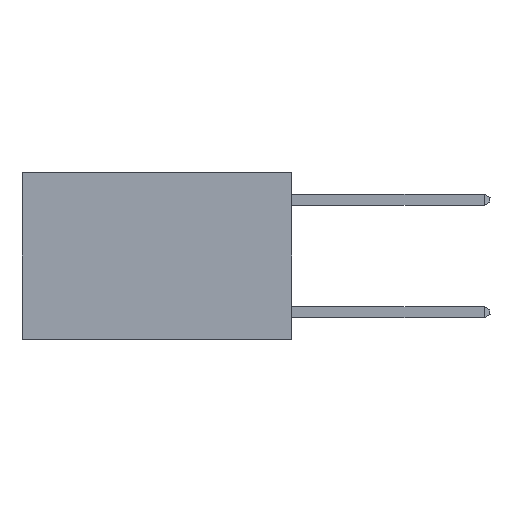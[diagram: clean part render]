
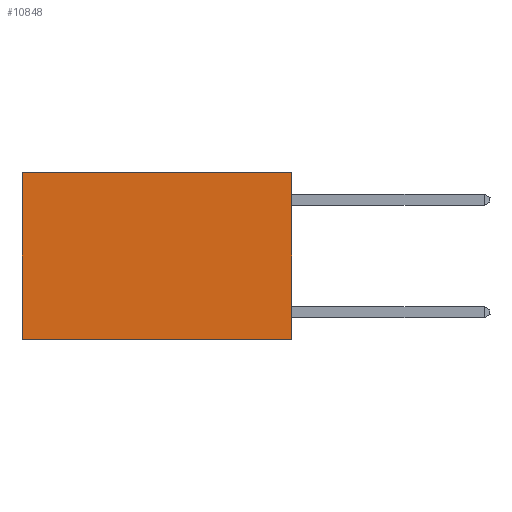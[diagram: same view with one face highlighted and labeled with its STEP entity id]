
A CAD part, left-side view. The second image highlights one B-rep face of the part: STEP entity #10848.
In plain terms, the highlighted planar face has unit normal (-1, 0, 0).
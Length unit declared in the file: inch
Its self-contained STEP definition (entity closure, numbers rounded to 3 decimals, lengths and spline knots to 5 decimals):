
#117 = ORIENTED_EDGE ( 'NONE', *, *, #21664, .F. ) ;
#2075 = CARTESIAN_POINT ( 'NONE',  ( 0.2625, 0.6, 0. ) ) ;
#2813 = LINE ( 'NONE', #24057, #13358 ) ;
#4246 = VECTOR ( 'NONE', #14963, 39.37008 ) ;
#4480 = VERTEX_POINT ( 'NONE', #2075 ) ;
#4677 = VERTEX_POINT ( 'NONE', #20266 ) ;
#7296 = EDGE_CURVE ( 'NONE', #13339, #4480, #17225, .T. ) ;
#7491 = FACE_OUTER_BOUND ( 'NONE', #22610, .T. ) ;
#9565 = ORIENTED_EDGE ( 'NONE', *, *, #13330, .F. ) ;
#10229 = ORIENTED_EDGE ( 'NONE', *, *, #18566, .T. ) ;
#10848 = ADVANCED_FACE ( 'NONE', ( #7491 ), #18692, .F. ) ;
#10866 = DIRECTION ( 'NONE',  ( 0., 0., -1. ) ) ;
#11054 = DIRECTION ( 'NONE',  ( 0., 0., -1. ) ) ;
#11266 = AXIS2_PLACEMENT_3D ( 'NONE', #12961, #22862, #11054 ) ;
#12796 = CARTESIAN_POINT ( 'NONE',  ( 0.2625, 0., -0.37 ) ) ;
#12961 = CARTESIAN_POINT ( 'NONE',  ( 0.2625, 0., 0. ) ) ;
#13027 = ORIENTED_EDGE ( 'NONE', *, *, #7296, .T. ) ;
#13203 = VECTOR ( 'NONE', #21121, 39.37008 ) ;
#13330 = EDGE_CURVE ( 'NONE', #13339, #24832, #2813, .T. ) ;
#13339 = VERTEX_POINT ( 'NONE', #23798 ) ;
#13358 = VECTOR ( 'NONE', #20010, 39.37008 ) ;
#14697 = LINE ( 'NONE', #20407, #19171 ) ;
#14963 = DIRECTION ( 'NONE',  ( 0., 1., 0. ) ) ;
#16854 = CARTESIAN_POINT ( 'NONE',  ( 0.2625, 0., 0. ) ) ;
#17076 = CARTESIAN_POINT ( 'NONE',  ( 0.2625, 0., -0.37 ) ) ;
#17225 = LINE ( 'NONE', #16854, #4246 ) ;
#18566 = EDGE_CURVE ( 'NONE', #4480, #4677, #14697, .T. ) ;
#18692 = PLANE ( 'NONE',  #11266 ) ;
#18722 = LINE ( 'NONE', #17076, #13203 ) ;
#19171 = VECTOR ( 'NONE', #10866, 39.37008 ) ;
#20010 = DIRECTION ( 'NONE',  ( 0., 0., -1. ) ) ;
#20266 = CARTESIAN_POINT ( 'NONE',  ( 0.2625, 0.6, -0.37 ) ) ;
#20407 = CARTESIAN_POINT ( 'NONE',  ( 0.2625, 0.6, 0. ) ) ;
#21121 = DIRECTION ( 'NONE',  ( 0., 1., 0. ) ) ;
#21664 = EDGE_CURVE ( 'NONE', #24832, #4677, #18722, .T. ) ;
#22610 = EDGE_LOOP ( 'NONE', ( #10229, #117, #9565, #13027 ) ) ;
#22862 = DIRECTION ( 'NONE',  ( 1., 0., 0. ) ) ;
#23798 = CARTESIAN_POINT ( 'NONE',  ( 0.2625, 0., 0. ) ) ;
#24057 = CARTESIAN_POINT ( 'NONE',  ( 0.2625, 0., 0. ) ) ;
#24832 = VERTEX_POINT ( 'NONE', #12796 ) ;
